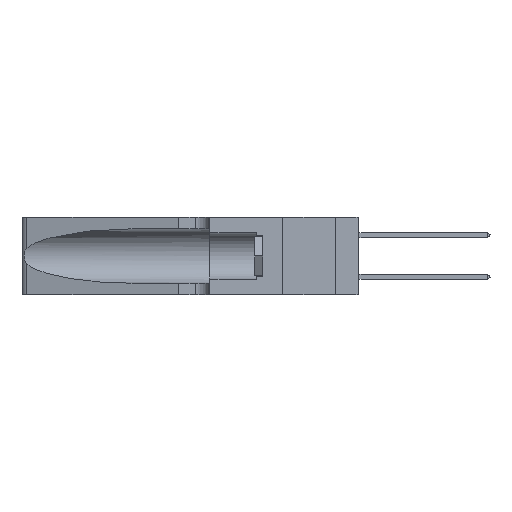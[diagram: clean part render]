
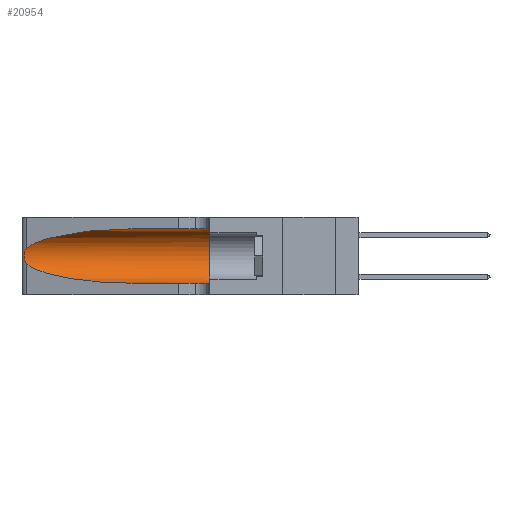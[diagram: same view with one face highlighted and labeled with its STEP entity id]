
A CAD part, left-side view. The second image highlights one B-rep face of the part: STEP entity #20954.
In plain terms, the highlighted cylindrical face has radius 3.308 mm (diameter 6.617 mm), a partial arc.
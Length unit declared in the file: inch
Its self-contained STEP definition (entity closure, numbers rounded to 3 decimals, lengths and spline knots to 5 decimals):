
#750 = CARTESIAN_POINT ( 'NONE',  ( 0.25639, 1.23184, 0.21858 ) ) ;
#910 = CARTESIAN_POINT ( 'NONE',  ( 0.26075, 1.23896, 0.19203 ) ) ;
#973 = EDGE_CURVE ( 'NONE', #37302, #21680, #7533, .T. ) ;
#3581 = EDGE_CURVE ( 'NONE', #14802, #31640, #5864, .T. ) ;
#4190 = CARTESIAN_POINT ( 'NONE',  ( 0.1305, 1.61858, 0.31525 ) ) ;
#4790 = CARTESIAN_POINT ( 'NONE',  ( 0.26017, 1.23833, 0.17102 ) ) ;
#5864 = LINE ( 'NONE', #16524, #24816 ) ;
#6976 = VERTEX_POINT ( 'NONE', #7380 ) ;
#7380 = CARTESIAN_POINT ( 'NONE',  ( 0.1305, 0.72297, 0.31525 ) ) ;
#7533 = B_SPLINE_CURVE_WITH_KNOTS ( 'NONE', 3,
 ( #42514, #15927, #750, #19896, #46230, #23679, #910, #27498, #4790, #31304, #8615, #35111, #12442, #38906 ),
 .UNSPECIFIED., .F., .F.,
 ( 4, 2, 2, 2, 2, 2, 4 ),
 ( 0., 0.00027, 0.00053, 0.00107, 0.0016, 0.00187, 0.00214 ),
 .UNSPECIFIED. ) ;
#7965 = CARTESIAN_POINT ( 'NONE',  ( 0.1305, 0.72297, 0.05475 ) ) ;
#8615 = CARTESIAN_POINT ( 'NONE',  ( 0.25789, 1.23486, 0.15765 ) ) ;
#9021 = DIRECTION ( 'NONE',  ( 0., -1., 0. ) ) ;
#9027 =( BOUNDED_CURVE ( )  B_SPLINE_CURVE ( 3, ( #26855, #45587, #30662, #7965 ),
 .UNSPECIFIED., .F., .F. ) 
 B_SPLINE_CURVE_WITH_KNOTS ( ( 4, 4 ),
 ( 3.44316, 4.71239 ),
 .UNSPECIFIED. ) 
 CURVE ( )  GEOMETRIC_REPRESENTATION_ITEM ( )  RATIONAL_B_SPLINE_CURVE ( ( 1., 0.87, 0.87, 1. ) ) 
 REPRESENTATION_ITEM ( '' )  );
#10872 = ORIENTED_EDGE ( 'NONE', *, *, #43803, .F. ) ;
#11243 = CARTESIAN_POINT ( 'NONE',  ( 0.25487, 1.22718, 0.22369 ) ) ;
#11346 = DIRECTION ( 'NONE',  ( 0., 1., 0. ) ) ;
#12442 = CARTESIAN_POINT ( 'NONE',  ( 0.25555, 1.22993, 0.14849 ) ) ;
#12592 = CARTESIAN_POINT ( 'NONE',  ( 0.1305, 0.35, 0.05475 ) ) ;
#12619 = CARTESIAN_POINT ( 'NONE',  ( 0.18966, 0.96281, 0.31525 ) ) ;
#12704 =( BOUNDED_CURVE ( )  B_SPLINE_CURVE ( 3, ( #35278, #12619, #39078, #16442 ),
 .UNSPECIFIED., .F., .F. ) 
 B_SPLINE_CURVE_WITH_KNOTS ( ( 4, 4 ),
 ( 1.5708, 2.84003 ),
 .UNSPECIFIED. ) 
 CURVE ( )  GEOMETRIC_REPRESENTATION_ITEM ( )  RATIONAL_B_SPLINE_CURVE ( ( 1., 0.87, 0.87, 1. ) ) 
 REPRESENTATION_ITEM ( '' )  );
#14083 = CARTESIAN_POINT ( 'NONE',  ( 0.1305, 1.61858, 0.185 ) ) ;
#14802 = VERTEX_POINT ( 'NONE', #33015 ) ;
#15927 = CARTESIAN_POINT ( 'NONE',  ( 0.25555, 1.22994, 0.2215 ) ) ;
#16009 = EDGE_CURVE ( 'NONE', #6976, #37302, #12704, .T. ) ;
#16442 = CARTESIAN_POINT ( 'NONE',  ( 0.25487, 1.22718, 0.22369 ) ) ;
#16524 = CARTESIAN_POINT ( 'NONE',  ( 0.1305, 1.61858, 0.05475 ) ) ;
#17340 = EDGE_LOOP ( 'NONE', ( #23874, #33969, #17408, #37508, #29818, #10872 ) ) ;
#17341 = CARTESIAN_POINT ( 'NONE',  ( 0.25487, 1.22718, 0.14631 ) ) ;
#17408 = ORIENTED_EDGE ( 'NONE', *, *, #46893, .T. ) ;
#19896 = CARTESIAN_POINT ( 'NONE',  ( 0.25787, 1.23484, 0.2124 ) ) ;
#20646 = LINE ( 'NONE', #4190, #39567 ) ;
#20674 = AXIS2_PLACEMENT_3D ( 'NONE', #14083, #47984, #36738 ) ;
#20954 = ADVANCED_FACE ( 'NONE', ( #40122 ), #38955, .F. ) ;
#21680 = VERTEX_POINT ( 'NONE', #17341 ) ;
#23061 = DIRECTION ( 'NONE',  ( 0., -1., 0. ) ) ;
#23679 = CARTESIAN_POINT ( 'NONE',  ( 0.26018, 1.23835, 0.19895 ) ) ;
#23874 = ORIENTED_EDGE ( 'NONE', *, *, #16009, .T. ) ;
#24816 = VECTOR ( 'NONE', #9021, 39.37008 ) ;
#26855 = CARTESIAN_POINT ( 'NONE',  ( 0.25487, 1.22718, 0.14631 ) ) ;
#27498 = CARTESIAN_POINT ( 'NONE',  ( 0.26075, 1.23896, 0.178 ) ) ;
#28870 = CARTESIAN_POINT ( 'NONE',  ( 0.1305, 0.35, 0.31525 ) ) ;
#29818 = ORIENTED_EDGE ( 'NONE', *, *, #39886, .F. ) ;
#30662 = CARTESIAN_POINT ( 'NONE',  ( 0.18966, 0.96281, 0.05475 ) ) ;
#31304 = CARTESIAN_POINT ( 'NONE',  ( 0.25856, 1.23593, 0.16098 ) ) ;
#31640 = VERTEX_POINT ( 'NONE', #12592 ) ;
#33015 = CARTESIAN_POINT ( 'NONE',  ( 0.1305, 0.72297, 0.05475 ) ) ;
#33969 = ORIENTED_EDGE ( 'NONE', *, *, #973, .T. ) ;
#34030 = CARTESIAN_POINT ( 'NONE',  ( 0.1305, 0.35, 0.185 ) ) ;
#35111 = CARTESIAN_POINT ( 'NONE',  ( 0.25639, 1.23186, 0.15144 ) ) ;
#35278 = CARTESIAN_POINT ( 'NONE',  ( 0.1305, 0.72297, 0.31525 ) ) ;
#36738 = DIRECTION ( 'NONE',  ( 0., 0., -1. ) ) ;
#37302 = VERTEX_POINT ( 'NONE', #11243 ) ;
#37508 = ORIENTED_EDGE ( 'NONE', *, *, #3581, .T. ) ;
#37823 = DIRECTION ( 'NONE',  ( 0., 0., 1. ) ) ;
#38906 = CARTESIAN_POINT ( 'NONE',  ( 0.25487, 1.22718, 0.14631 ) ) ;
#38955 = CYLINDRICAL_SURFACE ( 'NONE', #20674, 0.13025 ) ;
#39078 = CARTESIAN_POINT ( 'NONE',  ( 0.2373, 1.15595, 0.28018 ) ) ;
#39567 = VECTOR ( 'NONE', #23061, 39.37008 ) ;
#39886 = EDGE_CURVE ( 'NONE', #41646, #31640, #48668, .T. ) ;
#40122 = FACE_OUTER_BOUND ( 'NONE', #17340, .T. ) ;
#41646 = VERTEX_POINT ( 'NONE', #28870 ) ;
#42514 = CARTESIAN_POINT ( 'NONE',  ( 0.25487, 1.22718, 0.22369 ) ) ;
#43803 = EDGE_CURVE ( 'NONE', #6976, #41646, #20646, .T. ) ;
#45587 = CARTESIAN_POINT ( 'NONE',  ( 0.2373, 1.15595, 0.08982 ) ) ;
#46230 = CARTESIAN_POINT ( 'NONE',  ( 0.25854, 1.2359, 0.20912 ) ) ;
#46893 = EDGE_CURVE ( 'NONE', #21680, #14802, #9027, .T. ) ;
#47331 = AXIS2_PLACEMENT_3D ( 'NONE', #34030, #11346, #37823 ) ;
#47984 = DIRECTION ( 'NONE',  ( 0., -1., 0. ) ) ;
#48668 = CIRCLE ( 'NONE', #47331, 0.13025 ) ;
